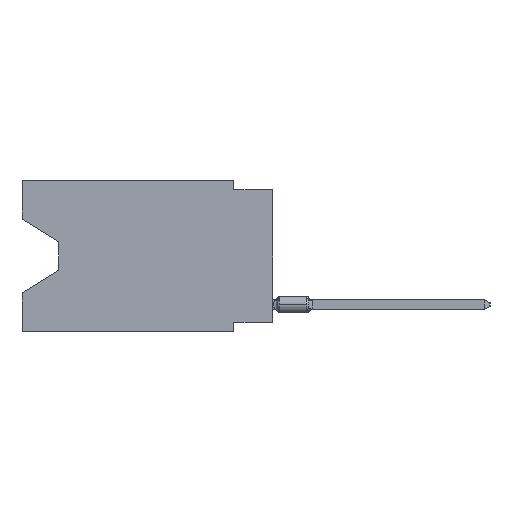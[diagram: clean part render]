
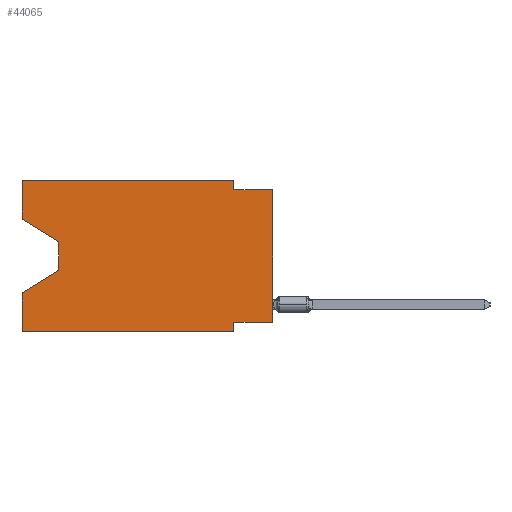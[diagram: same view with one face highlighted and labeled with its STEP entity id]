
A CAD part, left-side view. The second image highlights one B-rep face of the part: STEP entity #44065.
In plain terms, the highlighted planar face has unit normal (-1, 0, 0).
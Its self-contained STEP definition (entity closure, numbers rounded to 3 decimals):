
#2293 = LINE ( 'NONE', #72943, #70796 ) ;
#4045 = ORIENTED_EDGE ( 'NONE', *, *, #62828, .F. ) ;
#5761 = DIRECTION ( 'NONE',  ( 0., 0., 1. ) ) ;
#8425 = VERTEX_POINT ( 'NONE', #42845 ) ;
#8455 = EDGE_CURVE ( 'NONE', #54701, #60006, #11466, .T. ) ;
#9278 = DIRECTION ( 'NONE',  ( 0., 0., -1. ) ) ;
#10515 = PLANE ( 'NONE',  #45232 ) ;
#11007 = VERTEX_POINT ( 'NONE', #14833 ) ;
#11039 = DIRECTION ( 'NONE',  ( 0., 0., -1. ) ) ;
#11466 = LINE ( 'NONE', #61628, #23656 ) ;
#13220 = VECTOR ( 'NONE', #62480, 1000. ) ;
#14423 = EDGE_CURVE ( 'NONE', #34323, #62900, #76472, .T. ) ;
#14500 = VECTOR ( 'NONE', #5761, 1000. ) ;
#14797 = VERTEX_POINT ( 'NONE', #80172 ) ;
#14833 = CARTESIAN_POINT ( 'NONE',  ( 0., 2.54, 0. ) ) ;
#15826 = VERTEX_POINT ( 'NONE', #17919 ) ;
#16322 = VERTEX_POINT ( 'NONE', #45728 ) ;
#16748 = VECTOR ( 'NONE', #66964, 1000. ) ;
#17192 = LINE ( 'NONE', #54836, #16748 ) ;
#17919 = CARTESIAN_POINT ( 'NONE',  ( 0., 13.97, -4.013 ) ) ;
#18306 = LINE ( 'NONE', #57191, #14500 ) ;
#20438 = VECTOR ( 'NONE', #11039, 1000. ) ;
#20597 = DIRECTION ( 'NONE',  ( 0., -0.855, -0.519 ) ) ;
#20794 = EDGE_CURVE ( 'NONE', #15826, #39072, #35715, .T. ) ;
#21582 = CARTESIAN_POINT ( 'NONE',  ( 0., 2.54, -0.635 ) ) ;
#23656 = VECTOR ( 'NONE', #74186, 1000. ) ;
#25827 = ORIENTED_EDGE ( 'NONE', *, *, #20794, .T. ) ;
#27723 = LINE ( 'NONE', #39866, #78394 ) ;
#28580 = ORIENTED_EDGE ( 'NONE', *, *, #39080, .F. ) ;
#28933 = DIRECTION ( 'NONE',  ( 1., 0., 0. ) ) ;
#29073 = EDGE_CURVE ( 'NONE', #8425, #62900, #54827, .T. ) ;
#29821 = ORIENTED_EDGE ( 'NONE', *, *, #77747, .F. ) ;
#29904 = CARTESIAN_POINT ( 'NONE',  ( 0., 0., -0.635 ) ) ;
#30163 = CARTESIAN_POINT ( 'NONE',  ( 0., 0., 0. ) ) ;
#30603 = CARTESIAN_POINT ( 'NONE',  ( 0., 16.383, -7.36 ) ) ;
#31635 = VECTOR ( 'NONE', #62672, 1000. ) ;
#32742 = CARTESIAN_POINT ( 'NONE',  ( 0., 16.383, -2.546 ) ) ;
#34323 = VERTEX_POINT ( 'NONE', #21582 ) ;
#35715 = LINE ( 'NONE', #61193, #20438 ) ;
#35769 = CARTESIAN_POINT ( 'NONE',  ( 0., 2.54, -9.906 ) ) ;
#35779 = VECTOR ( 'NONE', #80556, 1000. ) ;
#37134 = ORIENTED_EDGE ( 'NONE', *, *, #14423, .F. ) ;
#37757 = ORIENTED_EDGE ( 'NONE', *, *, #76892, .F. ) ;
#39072 = VERTEX_POINT ( 'NONE', #49265 ) ;
#39080 = EDGE_CURVE ( 'NONE', #14797, #16322, #18306, .T. ) ;
#39866 = CARTESIAN_POINT ( 'NONE',  ( 0., 2.54, 0. ) ) ;
#42214 = CARTESIAN_POINT ( 'NONE',  ( 0., 0., -9.271 ) ) ;
#42845 = CARTESIAN_POINT ( 'NONE',  ( 0., 0., -9.271 ) ) ;
#44065 = ADVANCED_FACE ( 'NONE', ( #66959 ), #10515, .F. ) ;
#44905 = CARTESIAN_POINT ( 'NONE',  ( 0., 16.383, -9.906 ) ) ;
#45232 = AXIS2_PLACEMENT_3D ( 'NONE', #49384, #28933, #9278 ) ;
#45728 = CARTESIAN_POINT ( 'NONE',  ( 0., 16.383, 0. ) ) ;
#46958 = DIRECTION ( 'NONE',  ( 0., 0., -1. ) ) ;
#47755 = VERTEX_POINT ( 'NONE', #56686 ) ;
#47829 = EDGE_CURVE ( 'NONE', #54701, #76274, #2293, .T. ) ;
#48151 = DIRECTION ( 'NONE',  ( 0., 0., 1. ) ) ;
#48809 = LINE ( 'NONE', #82115, #35779 ) ;
#49265 = CARTESIAN_POINT ( 'NONE',  ( 0., 13.97, -5.893 ) ) ;
#49384 = CARTESIAN_POINT ( 'NONE',  ( 0., 16.383, 0. ) ) ;
#49470 = EDGE_CURVE ( 'NONE', #11007, #34323, #27723, .T. ) ;
#50361 = LINE ( 'NONE', #75042, #13220 ) ;
#52372 = LINE ( 'NONE', #32742, #80735 ) ;
#53030 = ORIENTED_EDGE ( 'NONE', *, *, #49470, .F. ) ;
#53867 = ORIENTED_EDGE ( 'NONE', *, *, #8455, .F. ) ;
#53980 = ORIENTED_EDGE ( 'NONE', *, *, #47829, .T. ) ;
#54418 = VECTOR ( 'NONE', #55566, 1000. ) ;
#54701 = VERTEX_POINT ( 'NONE', #44905 ) ;
#54827 = LINE ( 'NONE', #30163, #71551 ) ;
#54836 = CARTESIAN_POINT ( 'NONE',  ( 0., 16.383, 0. ) ) ;
#55566 = DIRECTION ( 'NONE',  ( 0., 1., 0. ) ) ;
#55975 = LINE ( 'NONE', #42214, #54418 ) ;
#56686 = CARTESIAN_POINT ( 'NONE',  ( 0., 2.54, -9.271 ) ) ;
#57191 = CARTESIAN_POINT ( 'NONE',  ( 0., 16.383, 0. ) ) ;
#58725 = EDGE_CURVE ( 'NONE', #14797, #15826, #52372, .T. ) ;
#60006 = VERTEX_POINT ( 'NONE', #30603 ) ;
#61193 = CARTESIAN_POINT ( 'NONE',  ( 0., 13.97, -4.013 ) ) ;
#61628 = CARTESIAN_POINT ( 'NONE',  ( 0., 16.383, 0. ) ) ;
#62480 = DIRECTION ( 'NONE',  ( 0., 0., -1. ) ) ;
#62672 = DIRECTION ( 'NONE',  ( 0., -1., 0. ) ) ;
#62828 = EDGE_CURVE ( 'NONE', #47755, #76274, #50361, .T. ) ;
#62900 = VERTEX_POINT ( 'NONE', #29904 ) ;
#62967 = ORIENTED_EDGE ( 'NONE', *, *, #58725, .T. ) ;
#65419 = DIRECTION ( 'NONE',  ( 0., -1., 0. ) ) ;
#65772 = ORIENTED_EDGE ( 'NONE', *, *, #82645, .T. ) ;
#66959 = FACE_OUTER_BOUND ( 'NONE', #67138, .T. ) ;
#66964 = DIRECTION ( 'NONE',  ( 0., -1., 0. ) ) ;
#67138 = EDGE_LOOP ( 'NONE', ( #62967, #25827, #65772, #53867, #53980, #4045, #37757, #80649, #37134, #53030, #29821, #28580 ) ) ;
#70796 = VECTOR ( 'NONE', #65419, 1000. ) ;
#71551 = VECTOR ( 'NONE', #48151, 1000. ) ;
#72943 = CARTESIAN_POINT ( 'NONE',  ( 0., 16.383, -9.906 ) ) ;
#74186 = DIRECTION ( 'NONE',  ( 0., 0., 1. ) ) ;
#75042 = CARTESIAN_POINT ( 'NONE',  ( 0., 2.54, -9.906 ) ) ;
#76058 = CARTESIAN_POINT ( 'NONE',  ( 0., 0., -0.635 ) ) ;
#76274 = VERTEX_POINT ( 'NONE', #35769 ) ;
#76472 = LINE ( 'NONE', #76058, #31635 ) ;
#76892 = EDGE_CURVE ( 'NONE', #8425, #47755, #55975, .T. ) ;
#77747 = EDGE_CURVE ( 'NONE', #16322, #11007, #17192, .T. ) ;
#78394 = VECTOR ( 'NONE', #46958, 1000. ) ;
#80172 = CARTESIAN_POINT ( 'NONE',  ( 0., 16.383, -2.546 ) ) ;
#80556 = DIRECTION ( 'NONE',  ( 0., 0.855, -0.519 ) ) ;
#80649 = ORIENTED_EDGE ( 'NONE', *, *, #29073, .T. ) ;
#80735 = VECTOR ( 'NONE', #20597, 1000. ) ;
#82115 = CARTESIAN_POINT ( 'NONE',  ( 0., 13.97, -5.893 ) ) ;
#82645 = EDGE_CURVE ( 'NONE', #39072, #60006, #48809, .T. ) ;
